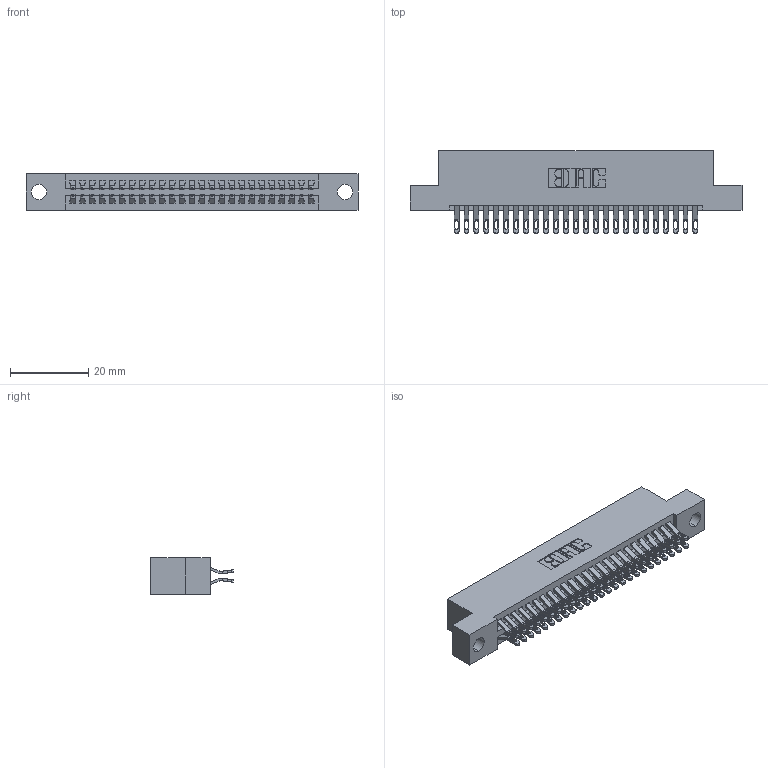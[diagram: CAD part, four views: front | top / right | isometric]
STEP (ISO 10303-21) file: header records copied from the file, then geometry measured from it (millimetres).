
FILE_DESCRIPTION (( 'STEP AP203' ), '1' );
FILE_NAME ('345-050-555-204.STEP', '2021-05-20T03:20:06', ( '' ), ( '' ), 'SwSTEP 2.0', 'SolidWorks 2020', '' );
FILE_SCHEMA (( 'CONFIG_CONTROL_DESIGN' ));
Length unit declared in the file: inch
Products named in the file (3): 345-292-001_555 Tail; 345-050-555-204; 345 Part_Flush Mounting Lugs - 0.156 Dia-TI
Assembly tree (51 placements, depth 2):
  345-050-555-204
    345 Part_Flush Mounting Lugs - 0.156 Dia-TI
    345-292-001_555 Tail  x50
Bounding box: 84.71 x 21.13 x 9.4 mm (x, y, z)
Volume: 8110 mm3; surface area: 12014.7 mm2
Topology: 51 solids, 51 shells, 2940 faces, 9227 edges, 6150 vertices
Faces by surface type: plane 1644, cylinder 1296
Entity records: 22649 total; most frequent: CARTESIAN_POINT 3852, ORIENTED_EDGE 3754, DIRECTION 3385, EDGE_CURVE 1877, LINE 1625, VECTOR 1625, VERTEX_POINT 1250, AXIS2_PLACEMENT_3D 880
